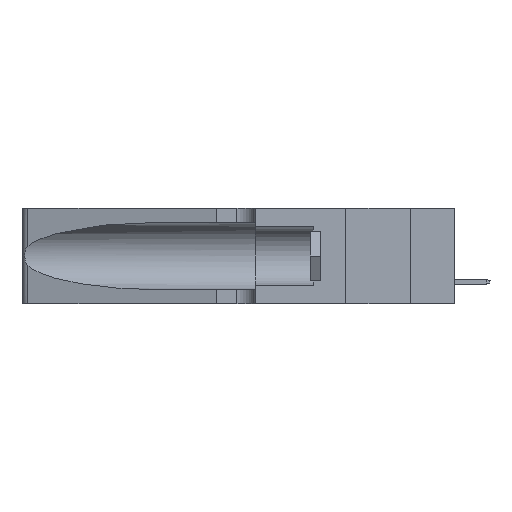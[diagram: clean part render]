
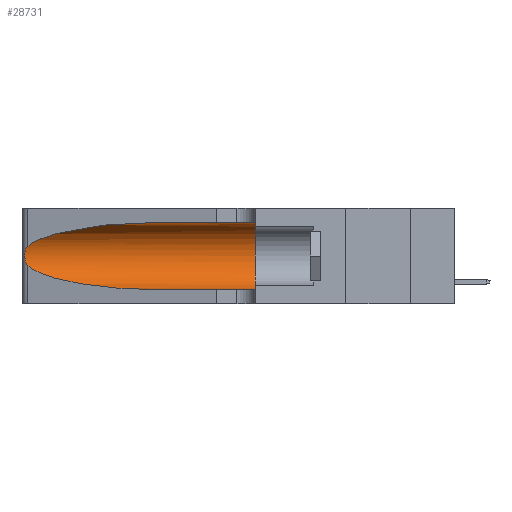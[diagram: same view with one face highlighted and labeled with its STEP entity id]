
A CAD part, left-side view. The second image highlights one B-rep face of the part: STEP entity #28731.
In plain terms, the highlighted cylindrical face has radius 3.308 mm (diameter 6.617 mm), a partial arc.
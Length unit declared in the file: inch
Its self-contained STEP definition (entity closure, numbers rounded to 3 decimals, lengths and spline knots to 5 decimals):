
#527 = CARTESIAN_POINT ( 'NONE',  ( 0.1305, 0.72297, 0.31525 ) ) ;
#1142 =( BOUNDED_CURVE ( )  B_SPLINE_CURVE ( 3, ( #22279, #35720, #33349, #21926 ),
 .UNSPECIFIED., .F., .T. ) 
 B_SPLINE_CURVE_WITH_KNOTS ( ( 4, 4 ),
 ( 3.44316, 4.71239 ),
 .UNSPECIFIED. ) 
 CURVE ( )  GEOMETRIC_REPRESENTATION_ITEM ( )  RATIONAL_B_SPLINE_CURVE ( ( 1., 0.87, 0.87, 1. ) ) 
 REPRESENTATION_ITEM ( '' )  );
#1164 = EDGE_CURVE ( 'NONE', #35347, #35358, #16552, .T. ) ;
#1973 = FACE_OUTER_BOUND ( 'NONE', #23501, .T. ) ;
#2754 = EDGE_CURVE ( 'NONE', #24298, #5003, #19085, .T. ) ;
#4146 = CARTESIAN_POINT ( 'NONE',  ( 0.1305, 0.72297, 0.05475 ) ) ;
#4652 = DIRECTION ( 'NONE',  ( 0., -1., 0. ) ) ;
#4671 = CARTESIAN_POINT ( 'NONE',  ( 0.26018, 1.23835, 0.19895 ) ) ;
#4861 = DIRECTION ( 'NONE',  ( 0., 0., -1. ) ) ;
#5003 = VERTEX_POINT ( 'NONE', #13936 ) ;
#5903 = CARTESIAN_POINT ( 'NONE',  ( 0.18966, 0.96281, 0.31525 ) ) ;
#7040 = CARTESIAN_POINT ( 'NONE',  ( 0.25555, 1.22993, 0.14849 ) ) ;
#7377 = LINE ( 'NONE', #21510, #29247 ) ;
#7587 = DIRECTION ( 'NONE',  ( 0., -1., 0. ) ) ;
#8378 = DIRECTION ( 'NONE',  ( 0., -1., 0. ) ) ;
#9303 = EDGE_CURVE ( 'NONE', #35347, #24298, #12255, .T. ) ;
#9916 = ORIENTED_EDGE ( 'NONE', *, *, #2754, .T. ) ;
#10102 = CARTESIAN_POINT ( 'NONE',  ( 0.25555, 1.22994, 0.2215 ) ) ;
#10153 = EDGE_CURVE ( 'NONE', #5003, #23924, #1142, .T. ) ;
#10323 = CARTESIAN_POINT ( 'NONE',  ( 0.1305, 0.72297, 0.31525 ) ) ;
#11177 = EDGE_CURVE ( 'NONE', #35358, #19293, #29731, .T. ) ;
#11821 = DIRECTION ( 'NONE',  ( 0., 1., 0. ) ) ;
#12255 =( BOUNDED_CURVE ( )  B_SPLINE_CURVE ( 3, ( #10323, #5903, #21563, #18839 ),
 .UNSPECIFIED., .F., .T. ) 
 B_SPLINE_CURVE_WITH_KNOTS ( ( 4, 4 ),
 ( 1.5708, 2.84003 ),
 .UNSPECIFIED. ) 
 CURVE ( )  GEOMETRIC_REPRESENTATION_ITEM ( )  RATIONAL_B_SPLINE_CURVE ( ( 1., 0.87, 0.87, 1. ) ) 
 REPRESENTATION_ITEM ( '' )  );
#12677 = CARTESIAN_POINT ( 'NONE',  ( 0.25854, 1.2359, 0.20912 ) ) ;
#13211 = CARTESIAN_POINT ( 'NONE',  ( 0.26017, 1.23833, 0.17102 ) ) ;
#13936 = CARTESIAN_POINT ( 'NONE',  ( 0.25487, 1.22718, 0.14631 ) ) ;
#14945 = ORIENTED_EDGE ( 'NONE', *, *, #1164, .F. ) ;
#15222 = ORIENTED_EDGE ( 'NONE', *, *, #9303, .T. ) ;
#15916 = CARTESIAN_POINT ( 'NONE',  ( 0.26075, 1.23896, 0.178 ) ) ;
#15929 = CARTESIAN_POINT ( 'NONE',  ( 0.1305, 1.61858, 0.185 ) ) ;
#16092 = CARTESIAN_POINT ( 'NONE',  ( 0.25487, 1.22718, 0.22369 ) ) ;
#16552 = LINE ( 'NONE', #35605, #26144 ) ;
#16964 = AXIS2_PLACEMENT_3D ( 'NONE', #22342, #11821, #22705 ) ;
#17358 = CARTESIAN_POINT ( 'NONE',  ( 0.1305, 0.35, 0.31525 ) ) ;
#18812 = CARTESIAN_POINT ( 'NONE',  ( 0.25639, 1.23184, 0.21858 ) ) ;
#18839 = CARTESIAN_POINT ( 'NONE',  ( 0.25487, 1.22718, 0.22369 ) ) ;
#19085 = B_SPLINE_CURVE_WITH_KNOTS ( 'NONE', 3,
 ( #16092, #10102, #18812, #31903, #12677, #4671, #29725, #15916, #13211, #24278, #35323, #23751, #7040, #34802 ),
 .UNSPECIFIED., .F., .F.,
 ( 4, 2, 2, 2, 2, 2, 4 ),
 ( 0., 0.00027, 0.00053, 0.00107, 0.0016, 0.00187, 0.00214 ),
 .UNSPECIFIED. ) ;
#19293 = VERTEX_POINT ( 'NONE', #32004 ) ;
#19934 = ORIENTED_EDGE ( 'NONE', *, *, #10153, .T. ) ;
#21510 = CARTESIAN_POINT ( 'NONE',  ( 0.1305, 1.61858, 0.05475 ) ) ;
#21563 = CARTESIAN_POINT ( 'NONE',  ( 0.2373, 1.15595, 0.28018 ) ) ;
#21926 = CARTESIAN_POINT ( 'NONE',  ( 0.1305, 0.72297, 0.05475 ) ) ;
#22279 = CARTESIAN_POINT ( 'NONE',  ( 0.25487, 1.22718, 0.14631 ) ) ;
#22342 = CARTESIAN_POINT ( 'NONE',  ( 0.1305, 0.35, 0.185 ) ) ;
#22705 = DIRECTION ( 'NONE',  ( 0., 0., 1. ) ) ;
#23501 = EDGE_LOOP ( 'NONE', ( #15222, #9916, #19934, #27397, #27088, #14945 ) ) ;
#23751 = CARTESIAN_POINT ( 'NONE',  ( 0.25639, 1.23186, 0.15144 ) ) ;
#23924 = VERTEX_POINT ( 'NONE', #4146 ) ;
#24278 = CARTESIAN_POINT ( 'NONE',  ( 0.25856, 1.23593, 0.16098 ) ) ;
#24298 = VERTEX_POINT ( 'NONE', #32598 ) ;
#24719 = AXIS2_PLACEMENT_3D ( 'NONE', #15929, #7587, #4861 ) ;
#26144 = VECTOR ( 'NONE', #8378, 39.37008 ) ;
#26813 = CYLINDRICAL_SURFACE ( 'NONE', #24719, 0.13025 ) ;
#27088 = ORIENTED_EDGE ( 'NONE', *, *, #11177, .F. ) ;
#27397 = ORIENTED_EDGE ( 'NONE', *, *, #30369, .T. ) ;
#28731 = ADVANCED_FACE ( 'NONE', ( #1973 ), #26813, .F. ) ;
#29247 = VECTOR ( 'NONE', #4652, 39.37008 ) ;
#29725 = CARTESIAN_POINT ( 'NONE',  ( 0.26075, 1.23896, 0.19203 ) ) ;
#29731 = CIRCLE ( 'NONE', #16964, 0.13025 ) ;
#30369 = EDGE_CURVE ( 'NONE', #23924, #19293, #7377, .T. ) ;
#31903 = CARTESIAN_POINT ( 'NONE',  ( 0.25787, 1.23484, 0.2124 ) ) ;
#32004 = CARTESIAN_POINT ( 'NONE',  ( 0.1305, 0.35, 0.05475 ) ) ;
#32598 = CARTESIAN_POINT ( 'NONE',  ( 0.25487, 1.22718, 0.22369 ) ) ;
#33349 = CARTESIAN_POINT ( 'NONE',  ( 0.18966, 0.96281, 0.05475 ) ) ;
#34802 = CARTESIAN_POINT ( 'NONE',  ( 0.25487, 1.22718, 0.14631 ) ) ;
#35323 = CARTESIAN_POINT ( 'NONE',  ( 0.25789, 1.23486, 0.15765 ) ) ;
#35347 = VERTEX_POINT ( 'NONE', #527 ) ;
#35358 = VERTEX_POINT ( 'NONE', #17358 ) ;
#35605 = CARTESIAN_POINT ( 'NONE',  ( 0.1305, 1.61858, 0.31525 ) ) ;
#35720 = CARTESIAN_POINT ( 'NONE',  ( 0.2373, 1.15595, 0.08982 ) ) ;
